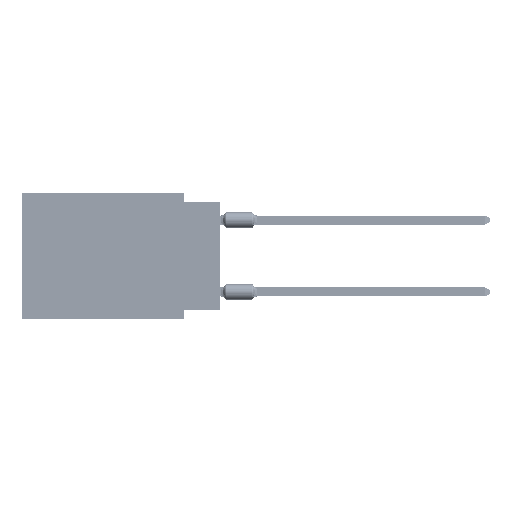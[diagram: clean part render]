
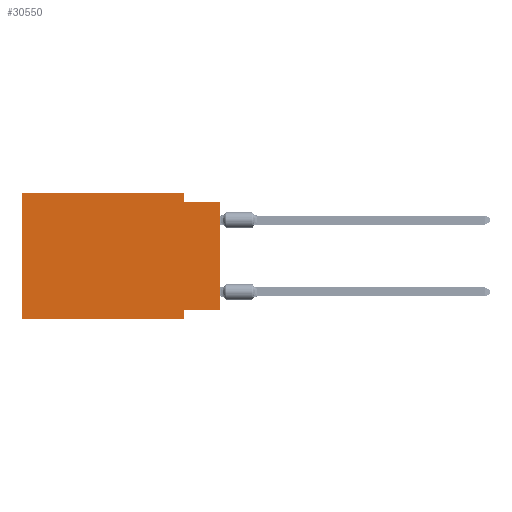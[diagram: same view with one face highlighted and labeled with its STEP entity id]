
A CAD part, left-side view. The second image highlights one B-rep face of the part: STEP entity #30550.
In plain terms, the highlighted planar face has unit normal (-1, 0, 0).
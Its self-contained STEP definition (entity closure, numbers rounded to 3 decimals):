
#12 = DIRECTION ( 'NONE',  ( 1., 0., 0. ) ) ;
#1708 = DIRECTION ( 'NONE',  ( 0., -1., 0. ) ) ;
#3655 = DIRECTION ( 'NONE',  ( 0., -1., 0. ) ) ;
#4806 = CARTESIAN_POINT ( 'NONE',  ( 0., 13.97, 0. ) ) ;
#6359 = ORIENTED_EDGE ( 'NONE', *, *, #43094, .F. ) ;
#7163 = ORIENTED_EDGE ( 'NONE', *, *, #47102, .F. ) ;
#8331 = CARTESIAN_POINT ( 'NONE',  ( 0., 13.97, 0. ) ) ;
#9365 = EDGE_CURVE ( 'NONE', #28208, #69294, #78138, .T. ) ;
#12317 = FACE_OUTER_BOUND ( 'NONE', #29920, .T. ) ;
#12654 = LINE ( 'NONE', #4806, #63008 ) ;
#12801 = DIRECTION ( 'NONE',  ( 0., 0., 1. ) ) ;
#14036 = ORIENTED_EDGE ( 'NONE', *, *, #32705, .T. ) ;
#14486 = CARTESIAN_POINT ( 'NONE',  ( 0., 0., -0.635 ) ) ;
#18702 = VERTEX_POINT ( 'NONE', #93884 ) ;
#18756 = VERTEX_POINT ( 'NONE', #47759 ) ;
#19867 = EDGE_CURVE ( 'NONE', #18702, #46303, #55124, .T. ) ;
#23151 = DIRECTION ( 'NONE',  ( 0., 0., -1. ) ) ;
#23779 = CARTESIAN_POINT ( 'NONE',  ( 0., 13.97, -8.89 ) ) ;
#25650 = CARTESIAN_POINT ( 'NONE',  ( 0., 2.54, -8.89 ) ) ;
#27544 = VECTOR ( 'NONE', #34740, 1000. ) ;
#28208 = VERTEX_POINT ( 'NONE', #92542 ) ;
#29446 = PLANE ( 'NONE',  #57902 ) ;
#29920 = EDGE_LOOP ( 'NONE', ( #77129, #74380, #73601, #92948, #6359, #14036, #39763, #7163 ) ) ;
#30550 = ADVANCED_FACE ( 'NONE', ( #12317 ), #29446, .F. ) ;
#30844 = CARTESIAN_POINT ( 'NONE',  ( 0., 2.54, 0. ) ) ;
#32705 = EDGE_CURVE ( 'NONE', #18756, #69294, #77246, .T. ) ;
#34342 = CARTESIAN_POINT ( 'NONE',  ( 0., 0., -8.255 ) ) ;
#34740 = DIRECTION ( 'NONE',  ( 0., 1., 0. ) ) ;
#35702 = VECTOR ( 'NONE', #50141, 1000. ) ;
#38221 = DIRECTION ( 'NONE',  ( 0., 0., -1. ) ) ;
#39763 = ORIENTED_EDGE ( 'NONE', *, *, #9365, .F. ) ;
#40696 = EDGE_CURVE ( 'NONE', #75860, #18702, #45699, .T. ) ;
#41538 = VECTOR ( 'NONE', #3655, 1000. ) ;
#42554 = DIRECTION ( 'NONE',  ( 0., -1., 0. ) ) ;
#43094 = EDGE_CURVE ( 'NONE', #18756, #79798, #48577, .T. ) ;
#45214 = CARTESIAN_POINT ( 'NONE',  ( 0., 2.54, 0. ) ) ;
#45699 = LINE ( 'NONE', #45214, #69201 ) ;
#46303 = VERTEX_POINT ( 'NONE', #14486 ) ;
#46497 = EDGE_CURVE ( 'NONE', #85981, #46303, #61003, .T. ) ;
#47102 = EDGE_CURVE ( 'NONE', #85981, #28208, #94102, .T. ) ;
#47759 = CARTESIAN_POINT ( 'NONE',  ( 0., 13.97, -8.89 ) ) ;
#48426 = CARTESIAN_POINT ( 'NONE',  ( 0., 2.54, -8.89 ) ) ;
#48577 = LINE ( 'NONE', #78532, #94594 ) ;
#50141 = DIRECTION ( 'NONE',  ( 0., 0., -1. ) ) ;
#50425 = CARTESIAN_POINT ( 'NONE',  ( 0., 0., -8.255 ) ) ;
#52008 = VECTOR ( 'NONE', #1708, 1000. ) ;
#55124 = LINE ( 'NONE', #86559, #41538 ) ;
#55579 = VECTOR ( 'NONE', #61488, 1000. ) ;
#57902 = AXIS2_PLACEMENT_3D ( 'NONE', #8331, #12, #38221 ) ;
#61003 = LINE ( 'NONE', #68857, #55579 ) ;
#61488 = DIRECTION ( 'NONE',  ( 0., 0., 1. ) ) ;
#63008 = VECTOR ( 'NONE', #42554, 1000. ) ;
#68857 = CARTESIAN_POINT ( 'NONE',  ( 0., 0., 0. ) ) ;
#69201 = VECTOR ( 'NONE', #23151, 1000. ) ;
#69294 = VERTEX_POINT ( 'NONE', #48426 ) ;
#69411 = EDGE_CURVE ( 'NONE', #79798, #75860, #12654, .T. ) ;
#73601 = ORIENTED_EDGE ( 'NONE', *, *, #40696, .F. ) ;
#74380 = ORIENTED_EDGE ( 'NONE', *, *, #19867, .F. ) ;
#75860 = VERTEX_POINT ( 'NONE', #30844 ) ;
#77129 = ORIENTED_EDGE ( 'NONE', *, *, #46497, .T. ) ;
#77246 = LINE ( 'NONE', #23779, #52008 ) ;
#78138 = LINE ( 'NONE', #25650, #35702 ) ;
#78532 = CARTESIAN_POINT ( 'NONE',  ( 0., 13.97, 0. ) ) ;
#79798 = VERTEX_POINT ( 'NONE', #90696 ) ;
#85981 = VERTEX_POINT ( 'NONE', #34342 ) ;
#86559 = CARTESIAN_POINT ( 'NONE',  ( 0., 0., -0.635 ) ) ;
#90696 = CARTESIAN_POINT ( 'NONE',  ( 0., 13.97, 0. ) ) ;
#92542 = CARTESIAN_POINT ( 'NONE',  ( 0., 2.54, -8.255 ) ) ;
#92948 = ORIENTED_EDGE ( 'NONE', *, *, #69411, .F. ) ;
#93884 = CARTESIAN_POINT ( 'NONE',  ( 0., 2.54, -0.635 ) ) ;
#94102 = LINE ( 'NONE', #50425, #27544 ) ;
#94594 = VECTOR ( 'NONE', #12801, 1000. ) ;
